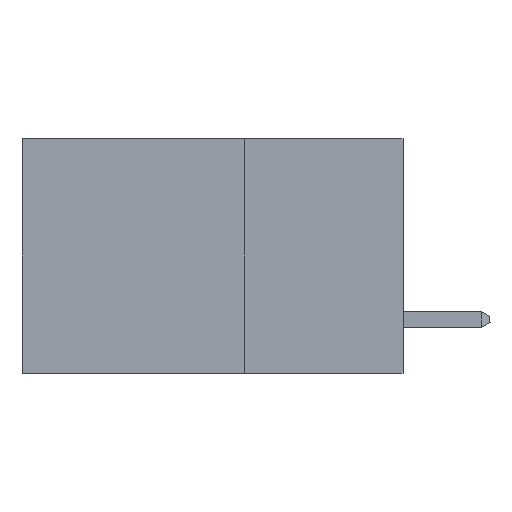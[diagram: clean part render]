
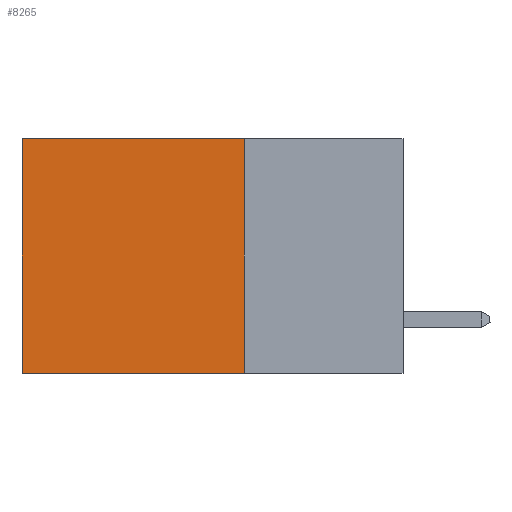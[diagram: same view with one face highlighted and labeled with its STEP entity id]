
A CAD part, left-side view. The second image highlights one B-rep face of the part: STEP entity #8265.
In plain terms, the highlighted planar face has unit normal (-1, 0, 0).
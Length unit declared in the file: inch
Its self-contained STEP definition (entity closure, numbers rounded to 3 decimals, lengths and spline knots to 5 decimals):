
#855 = EDGE_LOOP ( 'NONE', ( #3505, #4593, #6512, #32241 ) ) ;
#3505 = ORIENTED_EDGE ( 'NONE', *, *, #6718, .T. ) ;
#3811 = CARTESIAN_POINT ( 'NONE',  ( 0.2875, 0.25, -0.37 ) ) ;
#4593 = ORIENTED_EDGE ( 'NONE', *, *, #15803, .F. ) ;
#6512 = ORIENTED_EDGE ( 'NONE', *, *, #14828, .F. ) ;
#6718 = EDGE_CURVE ( 'NONE', #16885, #20759, #23653, .T. ) ;
#6780 = CARTESIAN_POINT ( 'NONE',  ( 0.2875, 0.25, -0.37 ) ) ;
#6870 = CARTESIAN_POINT ( 'NONE',  ( 0.2875, 0.25, 0. ) ) ;
#6919 = VECTOR ( 'NONE', #9954, 39.37008 ) ;
#8265 = ADVANCED_FACE ( 'NONE', ( #36615 ), #29534, .F. ) ;
#8947 = DIRECTION ( 'NONE',  ( 0., 0., -1. ) ) ;
#9954 = DIRECTION ( 'NONE',  ( 0., 1., 0. ) ) ;
#14828 = EDGE_CURVE ( 'NONE', #31235, #48757, #34942, .T. ) ;
#15803 = EDGE_CURVE ( 'NONE', #48757, #20759, #36700, .T. ) ;
#16549 = VECTOR ( 'NONE', #24965, 39.37008 ) ;
#16885 = VERTEX_POINT ( 'NONE', #43666 ) ;
#16946 = LINE ( 'NONE', #32486, #6919 ) ;
#19482 = DIRECTION ( 'NONE',  ( 0., 0., -1. ) ) ;
#20759 = VERTEX_POINT ( 'NONE', #28785 ) ;
#21593 = DIRECTION ( 'NONE',  ( 1., 0., 0. ) ) ;
#23653 = LINE ( 'NONE', #23842, #28983 ) ;
#23842 = CARTESIAN_POINT ( 'NONE',  ( 0.2875, 0.6, 0. ) ) ;
#24965 = DIRECTION ( 'NONE',  ( 0., 1., 0. ) ) ;
#28785 = CARTESIAN_POINT ( 'NONE',  ( 0.2875, 0.6, -0.37 ) ) ;
#28983 = VECTOR ( 'NONE', #19482, 39.37008 ) ;
#29295 = CARTESIAN_POINT ( 'NONE',  ( 0.2875, 0.25, 0. ) ) ;
#29534 = PLANE ( 'NONE',  #34490 ) ;
#30656 = CARTESIAN_POINT ( 'NONE',  ( 0.2875, 0.25, 0. ) ) ;
#31235 = VERTEX_POINT ( 'NONE', #30656 ) ;
#32241 = ORIENTED_EDGE ( 'NONE', *, *, #48461, .T. ) ;
#32486 = CARTESIAN_POINT ( 'NONE',  ( 0.2875, 0.25, 0. ) ) ;
#33357 = DIRECTION ( 'NONE',  ( 0., 0., -1. ) ) ;
#34490 = AXIS2_PLACEMENT_3D ( 'NONE', #6870, #21593, #33357 ) ;
#34942 = LINE ( 'NONE', #29295, #43747 ) ;
#36615 = FACE_OUTER_BOUND ( 'NONE', #855, .T. ) ;
#36700 = LINE ( 'NONE', #6780, #16549 ) ;
#43666 = CARTESIAN_POINT ( 'NONE',  ( 0.2875, 0.6, 0. ) ) ;
#43747 = VECTOR ( 'NONE', #8947, 39.37008 ) ;
#48461 = EDGE_CURVE ( 'NONE', #31235, #16885, #16946, .T. ) ;
#48757 = VERTEX_POINT ( 'NONE', #3811 ) ;
